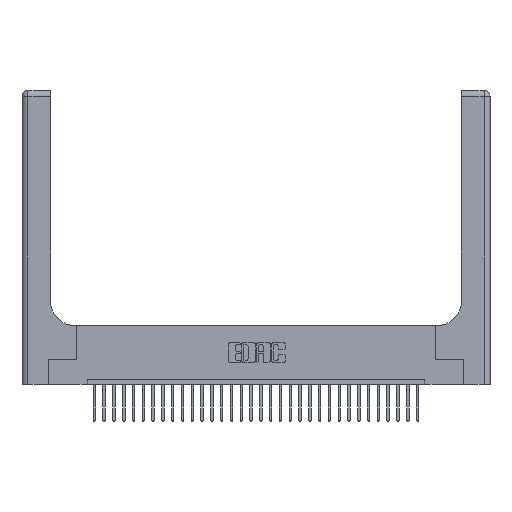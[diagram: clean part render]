
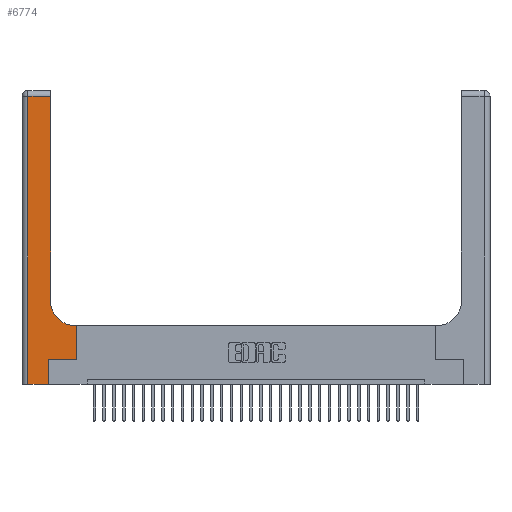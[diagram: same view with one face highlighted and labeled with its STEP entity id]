
A CAD part, top view. The second image highlights one B-rep face of the part: STEP entity #6774.
In plain terms, the highlighted planar face has unit normal (0, 0, 1).
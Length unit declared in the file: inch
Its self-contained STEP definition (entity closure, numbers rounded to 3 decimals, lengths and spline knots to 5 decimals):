
#419 = CARTESIAN_POINT ( 'NONE',  ( 0.5415, 0.85, 0.37 ) ) ;
#1068 = VERTEX_POINT ( 'NONE', #23731 ) ;
#1631 = DIRECTION ( 'NONE',  ( 0., -1., 0. ) ) ;
#1871 = DIRECTION ( 'NONE',  ( -1., 0., 0. ) ) ;
#2057 = ORIENTED_EDGE ( 'NONE', *, *, #17554, .T. ) ;
#2187 = LINE ( 'NONE', #15657, #25266 ) ;
#2393 = ORIENTED_EDGE ( 'NONE', *, *, #7647, .T. ) ;
#2579 = VERTEX_POINT ( 'NONE', #8637 ) ;
#2688 = VECTOR ( 'NONE', #24620, 39.37008 ) ;
#2912 = CARTESIAN_POINT ( 'NONE',  ( 0.06, 2.94, 0.37 ) ) ;
#3246 = PLANE ( 'NONE',  #27822 ) ;
#4029 = LINE ( 'NONE', #7459, #9781 ) ;
#4220 = VERTEX_POINT ( 'NONE', #2912 ) ;
#4395 = CARTESIAN_POINT ( 'NONE',  ( 0.2915, 0.85, 0.37 ) ) ;
#5308 = CARTESIAN_POINT ( 'NONE',  ( 0.5415, 0.6, 0.37 ) ) ;
#5715 = CARTESIAN_POINT ( 'NONE',  ( 0., 3., 0.37 ) ) ;
#5966 = DIRECTION ( 'NONE',  ( 1., 0., 0. ) ) ;
#6774 = ADVANCED_FACE ( 'NONE', ( #26733 ), #3246, .F. ) ;
#7064 = EDGE_CURVE ( 'NONE', #22443, #13223, #26152, .T. ) ;
#7077 = VECTOR ( 'NONE', #28861, 39.37008 ) ;
#7459 = CARTESIAN_POINT ( 'NONE',  ( 0.2915, 0.6, 0.37 ) ) ;
#7647 = EDGE_CURVE ( 'NONE', #24782, #20226, #11125, .T. ) ;
#7682 = ORIENTED_EDGE ( 'NONE', *, *, #15472, .T. ) ;
#8369 = ORIENTED_EDGE ( 'NONE', *, *, #24502, .T. ) ;
#8373 = VECTOR ( 'NONE', #11101, 39.37008 ) ;
#8637 = CARTESIAN_POINT ( 'NONE',  ( 0.269, 0.25, 0.37 ) ) ;
#9200 = ORIENTED_EDGE ( 'NONE', *, *, #26663, .T. ) ;
#9648 = ORIENTED_EDGE ( 'NONE', *, *, #23277, .T. ) ;
#9781 = VECTOR ( 'NONE', #1871, 39.37008 ) ;
#9840 = CARTESIAN_POINT ( 'NONE',  ( 0.269, 0., 0.37 ) ) ;
#11101 = DIRECTION ( 'NONE',  ( 0., 1., 0. ) ) ;
#11125 = CIRCLE ( 'NONE', #30951, 0.25 ) ;
#11662 = CARTESIAN_POINT ( 'NONE',  ( 0.269, 0., 0.37 ) ) ;
#12264 = LINE ( 'NONE', #18574, #31112 ) ;
#12317 = ORIENTED_EDGE ( 'NONE', *, *, #7064, .T. ) ;
#13199 = ORIENTED_EDGE ( 'NONE', *, *, #22577, .T. ) ;
#13223 = VERTEX_POINT ( 'NONE', #19752 ) ;
#13527 = EDGE_LOOP ( 'NONE', ( #7682, #13199, #9648, #8369, #9200, #23499, #12317, #2057, #2393 ) ) ;
#13683 = CARTESIAN_POINT ( 'NONE',  ( 0.2915, 3., 0.37 ) ) ;
#14335 = EDGE_CURVE ( 'NONE', #2579, #22443, #15390, .T. ) ;
#15390 = LINE ( 'NONE', #31638, #2688 ) ;
#15412 = VECTOR ( 'NONE', #1631, 39.37008 ) ;
#15472 = EDGE_CURVE ( 'NONE', #20226, #1068, #28808, .T. ) ;
#15657 = CARTESIAN_POINT ( 'NONE',  ( 0., 2.94, 0.37 ) ) ;
#15720 = DIRECTION ( 'NONE',  ( -1., 0., 0. ) ) ;
#17554 = EDGE_CURVE ( 'NONE', #13223, #24782, #4029, .T. ) ;
#18559 = DIRECTION ( 'NONE',  ( -1., 0., 0. ) ) ;
#18574 = CARTESIAN_POINT ( 'NONE',  ( 0., 0., 0.37 ) ) ;
#19752 = CARTESIAN_POINT ( 'NONE',  ( 0.5585, 0.6, 0.37 ) ) ;
#20226 = VERTEX_POINT ( 'NONE', #4395 ) ;
#20292 = CARTESIAN_POINT ( 'NONE',  ( 0.5585, 0.25, 0.37 ) ) ;
#20456 = DIRECTION ( 'NONE',  ( 1., 0., 0. ) ) ;
#21305 = VERTEX_POINT ( 'NONE', #29597 ) ;
#21348 = CARTESIAN_POINT ( 'NONE',  ( 0.06, 3., 0.37 ) ) ;
#22010 = LINE ( 'NONE', #21348, #15412 ) ;
#22443 = VERTEX_POINT ( 'NONE', #20292 ) ;
#22577 = EDGE_CURVE ( 'NONE', #1068, #4220, #2187, .T. ) ;
#23277 = EDGE_CURVE ( 'NONE', #4220, #21305, #22010, .T. ) ;
#23499 = ORIENTED_EDGE ( 'NONE', *, *, #14335, .T. ) ;
#23674 = DIRECTION ( 'NONE',  ( 0., 1., 0. ) ) ;
#23731 = CARTESIAN_POINT ( 'NONE',  ( 0.2915, 2.94, 0.37 ) ) ;
#24502 = EDGE_CURVE ( 'NONE', #21305, #26291, #12264, .T. ) ;
#24620 = DIRECTION ( 'NONE',  ( 1., 0., 0. ) ) ;
#24782 = VERTEX_POINT ( 'NONE', #5308 ) ;
#25266 = VECTOR ( 'NONE', #18559, 39.37008 ) ;
#26152 = LINE ( 'NONE', #30649, #29991 ) ;
#26291 = VERTEX_POINT ( 'NONE', #9840 ) ;
#26663 = EDGE_CURVE ( 'NONE', #26291, #2579, #31726, .T. ) ;
#26733 = FACE_OUTER_BOUND ( 'NONE', #13527, .T. ) ;
#27514 = DIRECTION ( 'NONE',  ( 0., 0., -1. ) ) ;
#27822 = AXIS2_PLACEMENT_3D ( 'NONE', #5715, #30345, #15720 ) ;
#28808 = LINE ( 'NONE', #13683, #8373 ) ;
#28861 = DIRECTION ( 'NONE',  ( 0., 1., 0. ) ) ;
#29597 = CARTESIAN_POINT ( 'NONE',  ( 0.06, 0., 0.37 ) ) ;
#29991 = VECTOR ( 'NONE', #23674, 39.37008 ) ;
#30345 = DIRECTION ( 'NONE',  ( 0., 0., -1. ) ) ;
#30649 = CARTESIAN_POINT ( 'NONE',  ( 0.5585, 0.25, 0.37 ) ) ;
#30951 = AXIS2_PLACEMENT_3D ( 'NONE', #419, #27514, #20456 ) ;
#31112 = VECTOR ( 'NONE', #5966, 39.37008 ) ;
#31638 = CARTESIAN_POINT ( 'NONE',  ( 0.269, 0.25, 0.37 ) ) ;
#31726 = LINE ( 'NONE', #11662, #7077 ) ;
